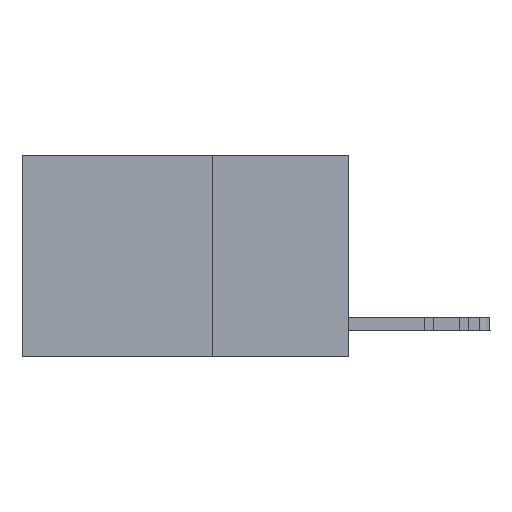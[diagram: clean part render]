
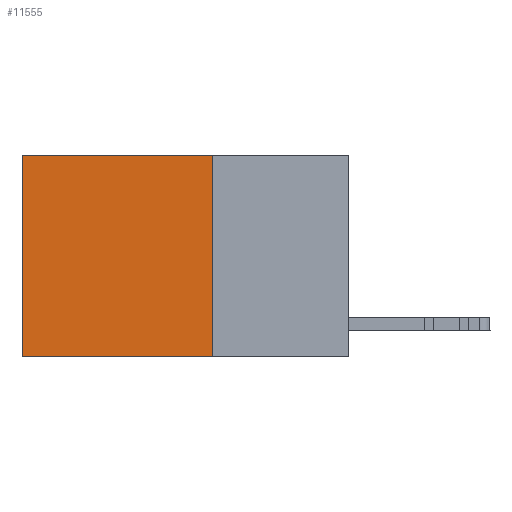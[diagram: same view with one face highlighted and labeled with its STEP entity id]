
A CAD part, left-side view. The second image highlights one B-rep face of the part: STEP entity #11555.
In plain terms, the highlighted planar face has unit normal (-1, 0, 0).
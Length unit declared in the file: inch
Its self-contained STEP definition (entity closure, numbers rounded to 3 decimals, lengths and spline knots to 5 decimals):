
#1215 = EDGE_CURVE ( 'NONE', #15100, #15613, #13424, .T. ) ;
#2280 = LINE ( 'NONE', #20573, #20427 ) ;
#3158 = CARTESIAN_POINT ( 'NONE',  ( 0.2625, 0.25, 0. ) ) ;
#3602 = VERTEX_POINT ( 'NONE', #3158 ) ;
#3829 = CARTESIAN_POINT ( 'NONE',  ( 0.2625, 0.6, 0. ) ) ;
#6254 = ORIENTED_EDGE ( 'NONE', *, *, #1215, .T. ) ;
#7852 = AXIS2_PLACEMENT_3D ( 'NONE', #11681, #23124, #15972 ) ;
#8205 = ORIENTED_EDGE ( 'NONE', *, *, #19616, .T. ) ;
#8235 = VERTEX_POINT ( 'NONE', #12106 ) ;
#9963 = LINE ( 'NONE', #21715, #27270 ) ;
#10524 = DIRECTION ( 'NONE',  ( 0., 1., 0. ) ) ;
#11380 = PLANE ( 'NONE',  #7852 ) ;
#11555 = ADVANCED_FACE ( 'NONE', ( #26048 ), #11380, .F. ) ;
#11681 = CARTESIAN_POINT ( 'NONE',  ( 0.2625, 0.25, 0. ) ) ;
#12106 = CARTESIAN_POINT ( 'NONE',  ( 0.2625, 0.25, -0.37 ) ) ;
#13424 = LINE ( 'NONE', #3829, #29116 ) ;
#15100 = VERTEX_POINT ( 'NONE', #22350 ) ;
#15613 = VERTEX_POINT ( 'NONE', #24785 ) ;
#15972 = DIRECTION ( 'NONE',  ( 0., 0., -1. ) ) ;
#18791 = LINE ( 'NONE', #28968, #25322 ) ;
#19616 = EDGE_CURVE ( 'NONE', #3602, #15100, #2280, .T. ) ;
#20251 = EDGE_CURVE ( 'NONE', #8235, #15613, #18791, .T. ) ;
#20427 = VECTOR ( 'NONE', #25443, 39.37008 ) ;
#20573 = CARTESIAN_POINT ( 'NONE',  ( 0.2625, 0.25, 0. ) ) ;
#20855 = EDGE_CURVE ( 'NONE', #3602, #8235, #9963, .T. ) ;
#21715 = CARTESIAN_POINT ( 'NONE',  ( 0.2625, 0.25, 0. ) ) ;
#22350 = CARTESIAN_POINT ( 'NONE',  ( 0.2625, 0.6, 0. ) ) ;
#23124 = DIRECTION ( 'NONE',  ( 1., 0., 0. ) ) ;
#23988 = DIRECTION ( 'NONE',  ( 0., 0., -1. ) ) ;
#24785 = CARTESIAN_POINT ( 'NONE',  ( 0.2625, 0.6, -0.37 ) ) ;
#25322 = VECTOR ( 'NONE', #10524, 39.37008 ) ;
#25420 = EDGE_LOOP ( 'NONE', ( #6254, #29047, #29611, #8205 ) ) ;
#25443 = DIRECTION ( 'NONE',  ( 0., 1., 0. ) ) ;
#26048 = FACE_OUTER_BOUND ( 'NONE', #25420, .T. ) ;
#27270 = VECTOR ( 'NONE', #23988, 39.37008 ) ;
#27442 = DIRECTION ( 'NONE',  ( 0., 0., -1. ) ) ;
#28968 = CARTESIAN_POINT ( 'NONE',  ( 0.2625, 0.25, -0.37 ) ) ;
#29047 = ORIENTED_EDGE ( 'NONE', *, *, #20251, .F. ) ;
#29116 = VECTOR ( 'NONE', #27442, 39.37008 ) ;
#29611 = ORIENTED_EDGE ( 'NONE', *, *, #20855, .F. ) ;
